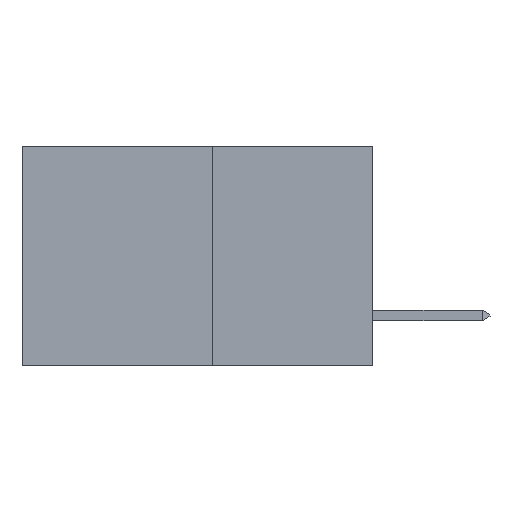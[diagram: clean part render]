
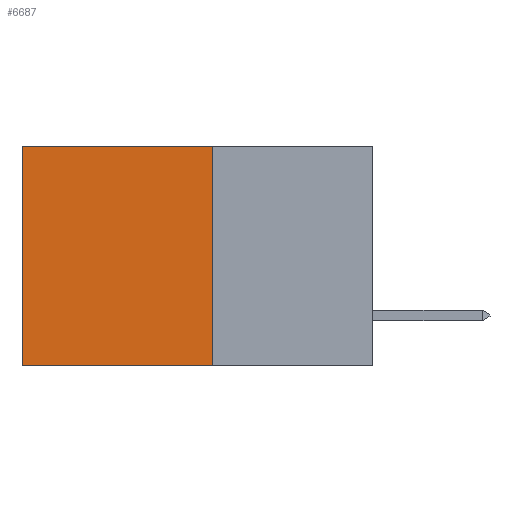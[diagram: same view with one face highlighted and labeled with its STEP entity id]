
A CAD part, left-side view. The second image highlights one B-rep face of the part: STEP entity #6687.
In plain terms, the highlighted planar face has unit normal (-1, 0, 0).
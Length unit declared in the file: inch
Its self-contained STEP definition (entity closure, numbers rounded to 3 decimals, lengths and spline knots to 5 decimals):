
#293 = EDGE_CURVE ( 'NONE', #2553, #2464, #5376, .T. ) ;
#419 = CARTESIAN_POINT ( 'NONE',  ( 0.277, 0.27, -0.37 ) ) ;
#652 = DIRECTION ( 'NONE',  ( 1., 0., 0. ) ) ;
#993 = DIRECTION ( 'NONE',  ( 0., 0., -1. ) ) ;
#1895 = EDGE_CURVE ( 'NONE', #10353, #2553, #9046, .T. ) ;
#2147 = VECTOR ( 'NONE', #7096, 39.37008 ) ;
#2197 = VECTOR ( 'NONE', #9515, 39.37008 ) ;
#2384 = FACE_OUTER_BOUND ( 'NONE', #3025, .T. ) ;
#2457 = CARTESIAN_POINT ( 'NONE',  ( 0.277, 0.27, -0.37 ) ) ;
#2464 = VERTEX_POINT ( 'NONE', #9441 ) ;
#2553 = VERTEX_POINT ( 'NONE', #9013 ) ;
#2675 = CARTESIAN_POINT ( 'NONE',  ( 0.277, 0.27, -0.37 ) ) ;
#2964 = LINE ( 'NONE', #2675, #7108 ) ;
#3025 = EDGE_LOOP ( 'NONE', ( #3752, #3582, #8351, #5186 ) ) ;
#3123 = VERTEX_POINT ( 'NONE', #2457 ) ;
#3537 = DIRECTION ( 'NONE',  ( 0., 1., 0. ) ) ;
#3582 = ORIENTED_EDGE ( 'NONE', *, *, #10585, .F. ) ;
#3752 = ORIENTED_EDGE ( 'NONE', *, *, #293, .T. ) ;
#4686 = CARTESIAN_POINT ( 'NONE',  ( 0.277, 0.27, 0. ) ) ;
#4727 = EDGE_CURVE ( 'NONE', #10353, #3123, #8734, .T. ) ;
#5126 = VECTOR ( 'NONE', #993, 39.37008 ) ;
#5186 = ORIENTED_EDGE ( 'NONE', *, *, #1895, .T. ) ;
#5376 = LINE ( 'NONE', #6590, #5126 ) ;
#5651 = CARTESIAN_POINT ( 'NONE',  ( 0.277, 0.27, -0.37 ) ) ;
#6443 = PLANE ( 'NONE',  #7251 ) ;
#6480 = DIRECTION ( 'NONE',  ( 0., 0., -1. ) ) ;
#6590 = CARTESIAN_POINT ( 'NONE',  ( 0.277, 0.59, -0.37 ) ) ;
#6687 = ADVANCED_FACE ( 'NONE', ( #2384 ), #6443, .F. ) ;
#6841 = CARTESIAN_POINT ( 'NONE',  ( 0.277, 0.27, 0. ) ) ;
#7096 = DIRECTION ( 'NONE',  ( 0., 0., -1. ) ) ;
#7108 = VECTOR ( 'NONE', #3537, 39.37008 ) ;
#7251 = AXIS2_PLACEMENT_3D ( 'NONE', #5651, #652, #6480 ) ;
#8351 = ORIENTED_EDGE ( 'NONE', *, *, #4727, .F. ) ;
#8734 = LINE ( 'NONE', #419, #2147 ) ;
#9013 = CARTESIAN_POINT ( 'NONE',  ( 0.277, 0.59, 0. ) ) ;
#9046 = LINE ( 'NONE', #6841, #2197 ) ;
#9441 = CARTESIAN_POINT ( 'NONE',  ( 0.277, 0.59, -0.37 ) ) ;
#9515 = DIRECTION ( 'NONE',  ( 0., 1., 0. ) ) ;
#10353 = VERTEX_POINT ( 'NONE', #4686 ) ;
#10585 = EDGE_CURVE ( 'NONE', #3123, #2464, #2964, .T. ) ;
